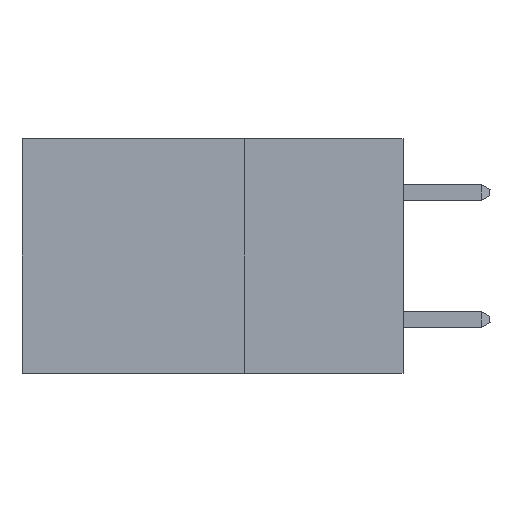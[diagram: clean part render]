
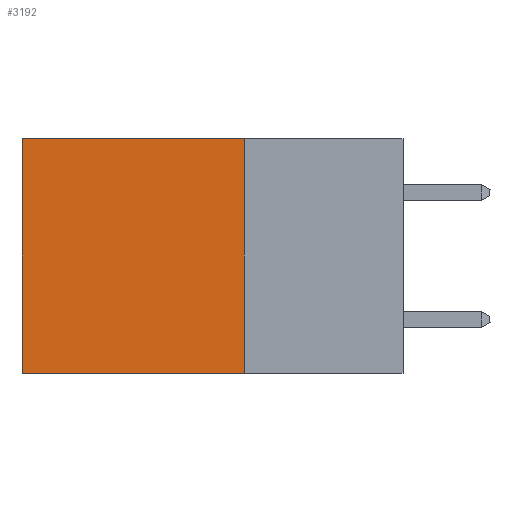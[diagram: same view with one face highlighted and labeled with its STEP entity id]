
A CAD part, left-side view. The second image highlights one B-rep face of the part: STEP entity #3192.
In plain terms, the highlighted planar face has unit normal (-1, 0, 0).
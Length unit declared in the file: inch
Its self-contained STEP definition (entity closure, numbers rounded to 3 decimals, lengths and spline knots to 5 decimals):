
#140 = EDGE_CURVE ( 'NONE', #19105, #4240, #24134, .T. ) ;
#832 = EDGE_CURVE ( 'NONE', #1343, #9378, #16529, .T. ) ;
#1017 = VECTOR ( 'NONE', #16407, 39.37008 ) ;
#1241 = PLANE ( 'NONE',  #16601 ) ;
#1343 = VERTEX_POINT ( 'NONE', #9421 ) ;
#1407 = LINE ( 'NONE', #3395, #2082 ) ;
#1704 = DIRECTION ( 'NONE',  ( 0., 0., -1. ) ) ;
#2082 = VECTOR ( 'NONE', #3493, 39.37008 ) ;
#3125 = VECTOR ( 'NONE', #1704, 39.37008 ) ;
#3192 = ADVANCED_FACE ( 'NONE', ( #23609 ), #1241, .F. ) ;
#3293 = ORIENTED_EDGE ( 'NONE', *, *, #832, .T. ) ;
#3395 = CARTESIAN_POINT ( 'NONE',  ( 0.2875, 0.25, 0. ) ) ;
#3493 = DIRECTION ( 'NONE',  ( 0., 1., 0. ) ) ;
#4240 = VERTEX_POINT ( 'NONE', #12453 ) ;
#7480 = ORIENTED_EDGE ( 'NONE', *, *, #140, .F. ) ;
#7722 = CARTESIAN_POINT ( 'NONE',  ( 0.2875, 0.6, 0. ) ) ;
#8564 = DIRECTION ( 'NONE',  ( 0., 1., 0. ) ) ;
#8846 = CARTESIAN_POINT ( 'NONE',  ( 0.2875, 0.25, 0. ) ) ;
#9378 = VERTEX_POINT ( 'NONE', #25043 ) ;
#9421 = CARTESIAN_POINT ( 'NONE',  ( 0.2875, 0.6, 0. ) ) ;
#9952 = DIRECTION ( 'NONE',  ( 0., 0., -1. ) ) ;
#10144 = VECTOR ( 'NONE', #8564, 39.37008 ) ;
#10229 = CARTESIAN_POINT ( 'NONE',  ( 0.2875, 0.25, 0. ) ) ;
#10497 = ORIENTED_EDGE ( 'NONE', *, *, #13561, .F. ) ;
#10551 = ORIENTED_EDGE ( 'NONE', *, *, #15033, .T. ) ;
#12453 = CARTESIAN_POINT ( 'NONE',  ( 0.2875, 0.25, -0.37 ) ) ;
#12485 = EDGE_LOOP ( 'NONE', ( #3293, #10497, #7480, #10551 ) ) ;
#13561 = EDGE_CURVE ( 'NONE', #4240, #9378, #24875, .T. ) ;
#14373 = CARTESIAN_POINT ( 'NONE',  ( 0.2875, 0.25, 0. ) ) ;
#15033 = EDGE_CURVE ( 'NONE', #19105, #1343, #1407, .T. ) ;
#16407 = DIRECTION ( 'NONE',  ( 0., 0., -1. ) ) ;
#16529 = LINE ( 'NONE', #7722, #1017 ) ;
#16601 = AXIS2_PLACEMENT_3D ( 'NONE', #14373, #23069, #9952 ) ;
#19105 = VERTEX_POINT ( 'NONE', #8846 ) ;
#21787 = CARTESIAN_POINT ( 'NONE',  ( 0.2875, 0.25, -0.37 ) ) ;
#23069 = DIRECTION ( 'NONE',  ( 1., 0., 0. ) ) ;
#23609 = FACE_OUTER_BOUND ( 'NONE', #12485, .T. ) ;
#24134 = LINE ( 'NONE', #10229, #3125 ) ;
#24875 = LINE ( 'NONE', #21787, #10144 ) ;
#25043 = CARTESIAN_POINT ( 'NONE',  ( 0.2875, 0.6, -0.37 ) ) ;
